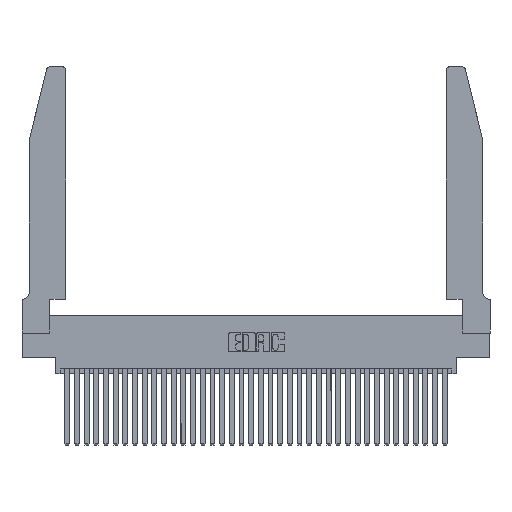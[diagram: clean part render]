
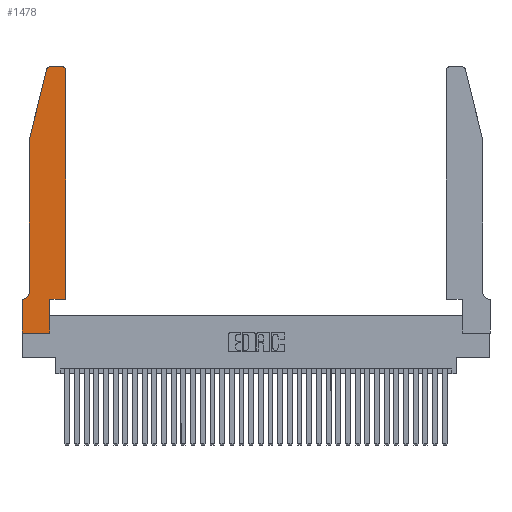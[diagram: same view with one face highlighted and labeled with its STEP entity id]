
A CAD part, top view. The second image highlights one B-rep face of the part: STEP entity #1478.
In plain terms, the highlighted planar face has unit normal (0, 0, 1).
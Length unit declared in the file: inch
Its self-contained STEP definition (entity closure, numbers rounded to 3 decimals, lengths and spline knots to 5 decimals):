
#16 = LINE ( 'NONE', #878, #13597 ) ;
#214 = CARTESIAN_POINT ( 'NONE',  ( 0.0755, 2., 0.37 ) ) ;
#257 = VERTEX_POINT ( 'NONE', #31453 ) ;
#629 = VERTEX_POINT ( 'NONE', #7815 ) ;
#878 = CARTESIAN_POINT ( 'NONE',  ( 0.0755, 2., 0.37 ) ) ;
#1349 = CARTESIAN_POINT ( 'NONE',  ( 0.4505, 0.35, 0.37 ) ) ;
#1478 = ADVANCED_FACE ( 'NONE', ( #17376 ), #2436, .T. ) ;
#1531 = VERTEX_POINT ( 'NONE', #8381 ) ;
#1657 = VECTOR ( 'NONE', #18464, 39.37008 ) ;
#2196 = ORIENTED_EDGE ( 'NONE', *, *, #12316, .T. ) ;
#2436 = PLANE ( 'NONE',  #17714 ) ;
#2709 = CARTESIAN_POINT ( 'NONE',  ( 0., 0.35, 0.37 ) ) ;
#3006 = ORIENTED_EDGE ( 'NONE', *, *, #10941, .T. ) ;
#3132 = EDGE_CURVE ( 'NONE', #1531, #629, #10282, .T. ) ;
#3195 = EDGE_CURVE ( 'NONE', #629, #15892, #35411, .T. ) ;
#3209 = CARTESIAN_POINT ( 'NONE',  ( 0.4205, 2.72, 0.37 ) ) ;
#3234 = DIRECTION ( 'NONE',  ( 0., -1., 0. ) ) ;
#3705 = VECTOR ( 'NONE', #31996, 39.37008 ) ;
#4130 = DIRECTION ( 'NONE',  ( 0., 0., 1. ) ) ;
#4530 = CIRCLE ( 'NONE', #6076, 0.03 ) ;
#5389 = DIRECTION ( 'NONE',  ( 0., 0., 1. ) ) ;
#6076 = AXIS2_PLACEMENT_3D ( 'NONE', #3209, #22967, #6104 ) ;
#6104 = DIRECTION ( 'NONE',  ( 1., 0., 0. ) ) ;
#6509 = EDGE_CURVE ( 'NONE', #21523, #18859, #21807, .T. ) ;
#6548 = DIRECTION ( 'NONE',  ( 1., 0., 0. ) ) ;
#7464 = CARTESIAN_POINT ( 'NONE',  ( 0.4505, 0.35, 0.37 ) ) ;
#7815 = CARTESIAN_POINT ( 'NONE',  ( 0.4505, 0.35, 0.37 ) ) ;
#8381 = CARTESIAN_POINT ( 'NONE',  ( 0.2865, 0.35, 0.37 ) ) ;
#8816 = AXIS2_PLACEMENT_3D ( 'NONE', #28255, #11631, #31013 ) ;
#9712 = CIRCLE ( 'NONE', #29800, 0.03 ) ;
#9758 = CARTESIAN_POINT ( 'NONE',  ( 0.2605, 2.75, 0.37 ) ) ;
#9789 = ORIENTED_EDGE ( 'NONE', *, *, #14111, .T. ) ;
#10282 = LINE ( 'NONE', #1349, #1657 ) ;
#10354 = DIRECTION ( 'NONE',  ( 0., 1., 0. ) ) ;
#10500 = VERTEX_POINT ( 'NONE', #26507 ) ;
#10941 = EDGE_CURVE ( 'NONE', #15892, #23105, #4530, .T. ) ;
#11315 = EDGE_LOOP ( 'NONE', ( #30819, #14046, #30974, #2196, #12782, #32555, #30928, #36292, #9789, #34950, #22879, #3006 ) ) ;
#11631 = DIRECTION ( 'NONE',  ( 0., 0., -1. ) ) ;
#11990 = CARTESIAN_POINT ( 'NONE',  ( 0.0055, 0.35, 0.37 ) ) ;
#12316 = EDGE_CURVE ( 'NONE', #12760, #257, #34976, .T. ) ;
#12760 = VERTEX_POINT ( 'NONE', #36042 ) ;
#12782 = ORIENTED_EDGE ( 'NONE', *, *, #16244, .T. ) ;
#13597 = VECTOR ( 'NONE', #29131, 39.37008 ) ;
#13663 = EDGE_CURVE ( 'NONE', #33122, #34436, #21613, .T. ) ;
#14046 = ORIENTED_EDGE ( 'NONE', *, *, #14336, .T. ) ;
#14111 = EDGE_CURVE ( 'NONE', #34436, #1531, #23298, .T. ) ;
#14336 = EDGE_CURVE ( 'NONE', #16875, #10500, #9712, .T. ) ;
#14340 = CARTESIAN_POINT ( 'NONE',  ( 0., 0., 0.37 ) ) ;
#15778 = EDGE_CURVE ( 'NONE', #10500, #12760, #16, .T. ) ;
#15892 = VERTEX_POINT ( 'NONE', #29593 ) ;
#16244 = EDGE_CURVE ( 'NONE', #257, #21523, #20991, .T. ) ;
#16875 = VERTEX_POINT ( 'NONE', #33636 ) ;
#17184 = DIRECTION ( 'NONE',  ( 0., 1., 0. ) ) ;
#17376 = FACE_OUTER_BOUND ( 'NONE', #11315, .T. ) ;
#17417 = VECTOR ( 'NONE', #33617, 39.37008 ) ;
#17714 = AXIS2_PLACEMENT_3D ( 'NONE', #19498, #5389, #25046 ) ;
#18121 = CARTESIAN_POINT ( 'NONE',  ( 0.2865, 0., 0.37 ) ) ;
#18282 = LINE ( 'NONE', #28084, #17417 ) ;
#18464 = DIRECTION ( 'NONE',  ( 1., 0., 0. ) ) ;
#18608 = VECTOR ( 'NONE', #3234, 39.37008 ) ;
#18859 = VERTEX_POINT ( 'NONE', #2709 ) ;
#19498 = CARTESIAN_POINT ( 'NONE',  ( 0., 0.35, 0.37 ) ) ;
#19685 = LINE ( 'NONE', #9758, #3705 ) ;
#20991 = CIRCLE ( 'NONE', #8816, 0.07 ) ;
#21065 = CARTESIAN_POINT ( 'NONE',  ( 0.284, 2.72, 0.37 ) ) ;
#21523 = VERTEX_POINT ( 'NONE', #11990 ) ;
#21613 = LINE ( 'NONE', #26185, #36208 ) ;
#21807 = LINE ( 'NONE', #22924, #29114 ) ;
#21982 = EDGE_CURVE ( 'NONE', #18859, #33122, #18282, .T. ) ;
#22879 = ORIENTED_EDGE ( 'NONE', *, *, #3195, .T. ) ;
#22924 = CARTESIAN_POINT ( 'NONE',  ( 0.0755, 0.35, 0.37 ) ) ;
#22967 = DIRECTION ( 'NONE',  ( 0., 0., 1. ) ) ;
#23105 = VERTEX_POINT ( 'NONE', #33432 ) ;
#23298 = LINE ( 'NONE', #28283, #36173 ) ;
#23850 = DIRECTION ( 'NONE',  ( 1., 0., 0. ) ) ;
#25046 = DIRECTION ( 'NONE',  ( 1., 0., 0. ) ) ;
#26185 = CARTESIAN_POINT ( 'NONE',  ( 0., 0., 0.37 ) ) ;
#26507 = CARTESIAN_POINT ( 'NONE',  ( 0.25487, 2.72718, 0.37 ) ) ;
#28084 = CARTESIAN_POINT ( 'NONE',  ( 0., 0., 0.37 ) ) ;
#28108 = VECTOR ( 'NONE', #10354, 39.37008 ) ;
#28255 = CARTESIAN_POINT ( 'NONE',  ( 0.0055, 0.42, 0.37 ) ) ;
#28283 = CARTESIAN_POINT ( 'NONE',  ( 0.2865, 0.35, 0.37 ) ) ;
#29114 = VECTOR ( 'NONE', #36110, 39.37008 ) ;
#29131 = DIRECTION ( 'NONE',  ( -0.239, -0.971, 0. ) ) ;
#29593 = CARTESIAN_POINT ( 'NONE',  ( 0.4505, 2.72, 0.37 ) ) ;
#29800 = AXIS2_PLACEMENT_3D ( 'NONE', #21065, #4130, #23850 ) ;
#30819 = ORIENTED_EDGE ( 'NONE', *, *, #32775, .T. ) ;
#30928 = ORIENTED_EDGE ( 'NONE', *, *, #21982, .T. ) ;
#30974 = ORIENTED_EDGE ( 'NONE', *, *, #15778, .T. ) ;
#31013 = DIRECTION ( 'NONE',  ( -1., 0., 0. ) ) ;
#31453 = CARTESIAN_POINT ( 'NONE',  ( 0.0755, 0.42, 0.37 ) ) ;
#31996 = DIRECTION ( 'NONE',  ( -1., 0., 0. ) ) ;
#32555 = ORIENTED_EDGE ( 'NONE', *, *, #6509, .T. ) ;
#32775 = EDGE_CURVE ( 'NONE', #23105, #16875, #19685, .T. ) ;
#33122 = VERTEX_POINT ( 'NONE', #14340 ) ;
#33432 = CARTESIAN_POINT ( 'NONE',  ( 0.4205, 2.75, 0.37 ) ) ;
#33617 = DIRECTION ( 'NONE',  ( 0., -1., 0. ) ) ;
#33636 = CARTESIAN_POINT ( 'NONE',  ( 0.284, 2.75, 0.37 ) ) ;
#34436 = VERTEX_POINT ( 'NONE', #18121 ) ;
#34950 = ORIENTED_EDGE ( 'NONE', *, *, #3132, .T. ) ;
#34976 = LINE ( 'NONE', #214, #18608 ) ;
#35411 = LINE ( 'NONE', #7464, #28108 ) ;
#36042 = CARTESIAN_POINT ( 'NONE',  ( 0.0755, 2., 0.37 ) ) ;
#36110 = DIRECTION ( 'NONE',  ( -1., 0., 0. ) ) ;
#36173 = VECTOR ( 'NONE', #17184, 39.37008 ) ;
#36208 = VECTOR ( 'NONE', #6548, 39.37008 ) ;
#36292 = ORIENTED_EDGE ( 'NONE', *, *, #13663, .T. ) ;
